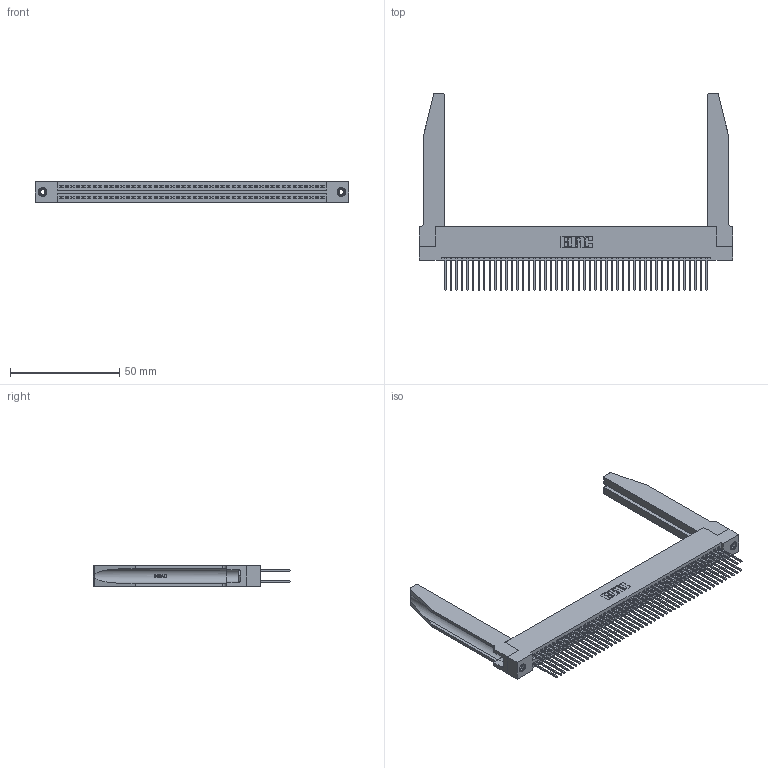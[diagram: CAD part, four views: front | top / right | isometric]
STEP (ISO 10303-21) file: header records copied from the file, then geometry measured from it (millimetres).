
FILE_DESCRIPTION (( 'STEP AP203' ), '1' );
FILE_NAME ('345-096-540-278.STEP', '2019-11-02T07:42:15', ( '' ), ( '' ), 'SwSTEP 2.0', 'SolidWorks 2016', '' );
FILE_SCHEMA (( 'CONFIG_CONTROL_DESIGN' ));
Length unit declared in the file: inch
Products named in the file (5): 345-220-078_345-220-078; 345-096-540-278; 345-250-001_345-250-001-102; 345 Part_Flush Mounting Lugs - 0.156 Dia-TH; 345-292-001_345-293-140
Assembly tree (101 placements, depth 2):
  345-096-540-278
    345 Part_Flush Mounting Lugs - 0.156 Dia-TH
    345-292-001_345-293-140  x96
    345-250-001_345-250-001-102  x2
    345-220-078_345-220-078  x2
Bounding box: 143.15 x 90.09 x 9.4 mm (x, y, z)
Volume: 22096.2 mm3; surface area: 29819 mm2
Topology: 101 solids, 101 shells, 5160 faces, 15253 edges, 10030 vertices
Faces by surface type: plane 3390, cylinder 1718, bspline 36, cone 12, torus 4
Entity records: 41612 total; most frequent: CARTESIAN_POINT 7887, ORIENTED_EDGE 6718, DIRECTION 5941, EDGE_CURVE 3359, LINE 2941, VECTOR 2941, VERTEX_POINT 2232, AXIS2_PLACEMENT_3D 1500
